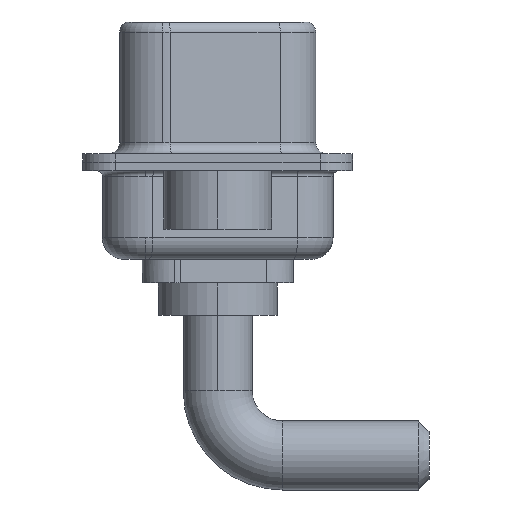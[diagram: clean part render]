
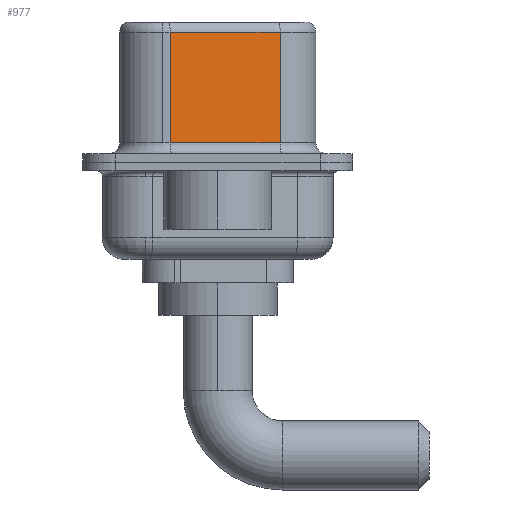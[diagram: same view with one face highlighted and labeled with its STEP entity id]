
A CAD part, left-side view. The second image highlights one B-rep face of the part: STEP entity #977.
In plain terms, the highlighted planar face has unit normal (-0.985, -0.174, 0).
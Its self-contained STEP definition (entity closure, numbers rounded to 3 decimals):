
#571 = VERTEX_POINT ( 'NONE', #6247 ) ;
#779 = LINE ( 'NONE', #3101, #14239 ) ;
#977 = ADVANCED_FACE ( 'NONE', ( #1226 ), #13306, .F. ) ;
#1205 = EDGE_LOOP ( 'NONE', ( #8028, #14875, #13523, #12732 ) ) ;
#1226 = FACE_OUTER_BOUND ( 'NONE', #1205, .T. ) ;
#1314 = CARTESIAN_POINT ( 'NONE',  ( 4.555, -2.897, 6.52 ) ) ;
#1827 = DIRECTION ( 'NONE',  ( 0., 0., -1. ) ) ;
#2344 = CARTESIAN_POINT ( 'NONE',  ( 4.555, -2.897, 6.02 ) ) ;
#2890 = VECTOR ( 'NONE', #14414, 1000. ) ;
#3101 = CARTESIAN_POINT ( 'NONE',  ( 3.655, 2.203, 6.52 ) ) ;
#3694 = CARTESIAN_POINT ( 'NONE',  ( 4.555, -2.897, 6.52 ) ) ;
#3767 = DIRECTION ( 'NONE',  ( 0.985, 0.174, 0. ) ) ;
#4864 = CARTESIAN_POINT ( 'NONE',  ( 4.555, -2.897, 6.02 ) ) ;
#5240 = VECTOR ( 'NONE', #8212, 1000. ) ;
#5501 = EDGE_CURVE ( 'NONE', #7524, #571, #8282, .T. ) ;
#6247 = CARTESIAN_POINT ( 'NONE',  ( 4.555, -2.897, 0.9 ) ) ;
#6289 = AXIS2_PLACEMENT_3D ( 'NONE', #3694, #3767, #9790 ) ;
#7524 = VERTEX_POINT ( 'NONE', #14376 ) ;
#8028 = ORIENTED_EDGE ( 'NONE', *, *, #14870, .F. ) ;
#8212 = DIRECTION ( 'NONE',  ( -0.174, 0.985, 0. ) ) ;
#8282 = LINE ( 'NONE', #9554, #2890 ) ;
#9554 = CARTESIAN_POINT ( 'NONE',  ( 4.555, -2.897, 0.9 ) ) ;
#9790 = DIRECTION ( 'NONE',  ( -0.174, 0.985, 0. ) ) ;
#10290 = EDGE_CURVE ( 'NONE', #11057, #13894, #11871, .T. ) ;
#10988 = LINE ( 'NONE', #1314, #14227 ) ;
#11057 = VERTEX_POINT ( 'NONE', #4864 ) ;
#11450 = CARTESIAN_POINT ( 'NONE',  ( 3.655, 2.203, 6.02 ) ) ;
#11871 = LINE ( 'NONE', #2344, #5240 ) ;
#12732 = ORIENTED_EDGE ( 'NONE', *, *, #5501, .T. ) ;
#13306 = PLANE ( 'NONE',  #6289 ) ;
#13394 = DIRECTION ( 'NONE',  ( 0., 0., -1. ) ) ;
#13523 = ORIENTED_EDGE ( 'NONE', *, *, #15459, .T. ) ;
#13894 = VERTEX_POINT ( 'NONE', #11450 ) ;
#14227 = VECTOR ( 'NONE', #13394, 1000. ) ;
#14239 = VECTOR ( 'NONE', #1827, 1000. ) ;
#14376 = CARTESIAN_POINT ( 'NONE',  ( 3.655, 2.203, 0.9 ) ) ;
#14414 = DIRECTION ( 'NONE',  ( 0.174, -0.985, 0. ) ) ;
#14870 = EDGE_CURVE ( 'NONE', #11057, #571, #10988, .T. ) ;
#14875 = ORIENTED_EDGE ( 'NONE', *, *, #10290, .T. ) ;
#15459 = EDGE_CURVE ( 'NONE', #13894, #7524, #779, .T. ) ;
